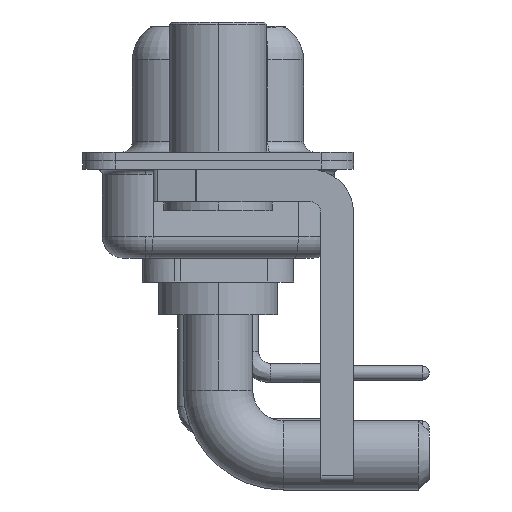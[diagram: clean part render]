
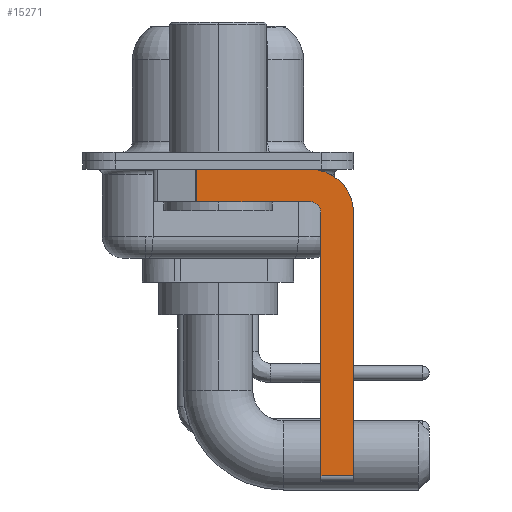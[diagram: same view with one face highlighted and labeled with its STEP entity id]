
A CAD part, left-side view. The second image highlights one B-rep face of the part: STEP entity #15271.
In plain terms, the highlighted planar face has unit normal (-1, 0, 0).
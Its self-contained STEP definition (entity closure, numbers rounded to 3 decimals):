
#311 = DIRECTION ( 'NONE',  ( 0., 0., -1. ) ) ;
#549 = VERTEX_POINT ( 'NONE', #6523 ) ;
#1075 = AXIS2_PLACEMENT_3D ( 'NONE', #1926, #17309, #311 ) ;
#1120 = VERTEX_POINT ( 'NONE', #7092 ) ;
#1289 = EDGE_CURVE ( 'NONE', #5336, #549, #20983, .T. ) ;
#1688 = ORIENTED_EDGE ( 'NONE', *, *, #20255, .F. ) ;
#1798 = VERTEX_POINT ( 'NONE', #9881 ) ;
#1926 = CARTESIAN_POINT ( 'NONE',  ( -2.9, -4.25, -2.4 ) ) ;
#3074 = EDGE_CURVE ( 'NONE', #5880, #23996, #4614, .T. ) ;
#3326 = DIRECTION ( 'NONE',  ( 0., -1., 0. ) ) ;
#3862 = EDGE_CURVE ( 'NONE', #11343, #1120, #5837, .T. ) ;
#3951 = CARTESIAN_POINT ( 'NONE',  ( -2.9, -6.25, -2.4 ) ) ;
#4060 = VECTOR ( 'NONE', #6453, 1000. ) ;
#4614 = CIRCLE ( 'NONE', #1075, 2. ) ;
#4810 = CARTESIAN_POINT ( 'NONE',  ( -2.9, -4.25, -1.9 ) ) ;
#5336 = VERTEX_POINT ( 'NONE', #12041 ) ;
#5642 = DIRECTION ( 'NONE',  ( -1., 0., 0. ) ) ;
#5837 = LINE ( 'NONE', #9552, #8067 ) ;
#5880 = VERTEX_POINT ( 'NONE', #12763 ) ;
#6453 = DIRECTION ( 'NONE',  ( 0., -1., 0. ) ) ;
#6523 = CARTESIAN_POINT ( 'NONE',  ( -2.9, -4.75, -2.4 ) ) ;
#6534 = LINE ( 'NONE', #14611, #13348 ) ;
#6840 = EDGE_LOOP ( 'NONE', ( #9832, #13648, #16770, #1688, #8673, #15106, #12919, #22805 ) ) ;
#7074 = VECTOR ( 'NONE', #17632, 1000. ) ;
#7092 = CARTESIAN_POINT ( 'NONE',  ( -2.9, 0.978, -1.9 ) ) ;
#7145 = DIRECTION ( 'NONE',  ( 1., 0., 0. ) ) ;
#7941 = DIRECTION ( 'NONE',  ( 0., 1., 0. ) ) ;
#8067 = VECTOR ( 'NONE', #7941, 1000. ) ;
#8509 = FACE_OUTER_BOUND ( 'NONE', #6840, .T. ) ;
#8673 = ORIENTED_EDGE ( 'NONE', *, *, #1289, .F. ) ;
#9001 = CARTESIAN_POINT ( 'NONE',  ( -2.9, -4.25, -2.4 ) ) ;
#9326 = EDGE_CURVE ( 'NONE', #5336, #1798, #6534, .T. ) ;
#9408 = DIRECTION ( 'NONE',  ( 0., 0., -1. ) ) ;
#9552 = CARTESIAN_POINT ( 'NONE',  ( -2.9, -4.25, -1.9 ) ) ;
#9777 = CARTESIAN_POINT ( 'NONE',  ( -2.9, -6.25, -2.4 ) ) ;
#9832 = ORIENTED_EDGE ( 'NONE', *, *, #23624, .F. ) ;
#9881 = CARTESIAN_POINT ( 'NONE',  ( -2.9, -6.25, -14.55 ) ) ;
#10499 = DIRECTION ( 'NONE',  ( 0., 0., -1. ) ) ;
#11126 = EDGE_CURVE ( 'NONE', #23996, #1798, #18963, .T. ) ;
#11343 = VERTEX_POINT ( 'NONE', #4810 ) ;
#12041 = CARTESIAN_POINT ( 'NONE',  ( -2.9, -4.75, -14.55 ) ) ;
#12427 = CARTESIAN_POINT ( 'NONE',  ( -2.9, 3., -0.4 ) ) ;
#12763 = CARTESIAN_POINT ( 'NONE',  ( -2.9, -4.25, -0.4 ) ) ;
#12824 = DIRECTION ( 'NONE',  ( 0., 0., -1. ) ) ;
#12919 = ORIENTED_EDGE ( 'NONE', *, *, #11126, .F. ) ;
#13348 = VECTOR ( 'NONE', #3326, 1000. ) ;
#13420 = CARTESIAN_POINT ( 'NONE',  ( -2.9, -4.75, -14.8 ) ) ;
#13648 = ORIENTED_EDGE ( 'NONE', *, *, #17652, .T. ) ;
#13813 = VERTEX_POINT ( 'NONE', #18418 ) ;
#14163 = LINE ( 'NONE', #21729, #15884 ) ;
#14611 = CARTESIAN_POINT ( 'NONE',  ( -2.9, -4.25, -14.55 ) ) ;
#15002 = AXIS2_PLACEMENT_3D ( 'NONE', #9001, #7145, #10499 ) ;
#15106 = ORIENTED_EDGE ( 'NONE', *, *, #9326, .T. ) ;
#15271 = ADVANCED_FACE ( 'NONE', ( #8509 ), #20316, .F. ) ;
#15884 = VECTOR ( 'NONE', #12824, 1000. ) ;
#16770 = ORIENTED_EDGE ( 'NONE', *, *, #3862, .F. ) ;
#17309 = DIRECTION ( 'NONE',  ( 1., 0., 0. ) ) ;
#17632 = DIRECTION ( 'NONE',  ( 0., 0., 1. ) ) ;
#17652 = EDGE_CURVE ( 'NONE', #13813, #1120, #14163, .T. ) ;
#18418 = CARTESIAN_POINT ( 'NONE',  ( -2.9, 0.978, -0.4 ) ) ;
#18963 = LINE ( 'NONE', #3951, #23294 ) ;
#19881 = AXIS2_PLACEMENT_3D ( 'NONE', #22639, #5642, #20899 ) ;
#20255 = EDGE_CURVE ( 'NONE', #549, #11343, #20695, .T. ) ;
#20316 = PLANE ( 'NONE',  #15002 ) ;
#20695 = CIRCLE ( 'NONE', #19881, 0.5 ) ;
#20899 = DIRECTION ( 'NONE',  ( 0., 0., 1. ) ) ;
#20983 = LINE ( 'NONE', #13420, #7074 ) ;
#21729 = CARTESIAN_POINT ( 'NONE',  ( -2.9, 0.978, -1.9 ) ) ;
#22639 = CARTESIAN_POINT ( 'NONE',  ( -2.9, -4.25, -2.4 ) ) ;
#22805 = ORIENTED_EDGE ( 'NONE', *, *, #3074, .F. ) ;
#23294 = VECTOR ( 'NONE', #9408, 1000. ) ;
#23486 = LINE ( 'NONE', #12427, #4060 ) ;
#23624 = EDGE_CURVE ( 'NONE', #13813, #5880, #23486, .T. ) ;
#23996 = VERTEX_POINT ( 'NONE', #9777 ) ;
